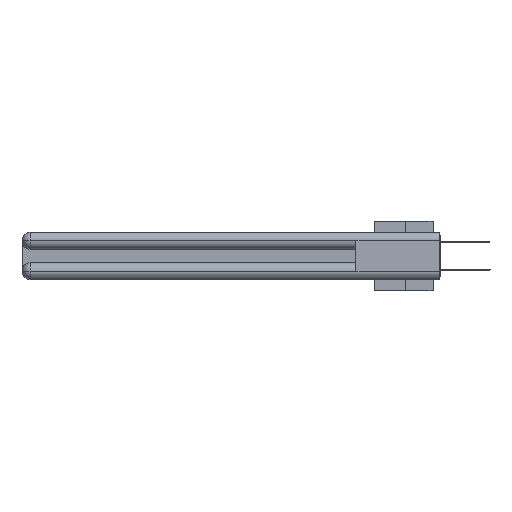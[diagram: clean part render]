
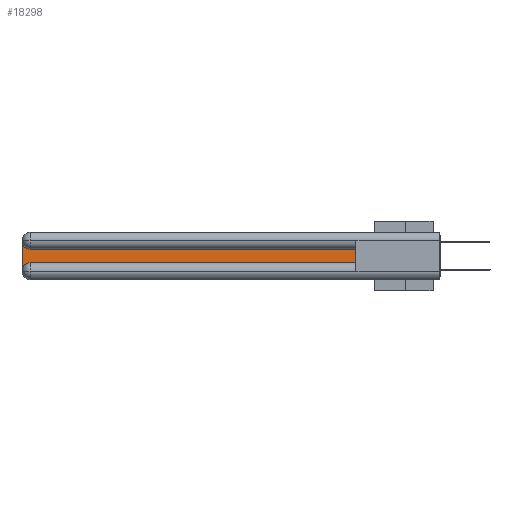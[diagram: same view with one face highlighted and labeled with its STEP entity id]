
A CAD part, left-side view. The second image highlights one B-rep face of the part: STEP entity #18298.
In plain terms, the highlighted planar face has unit normal (-1, 0, 0).
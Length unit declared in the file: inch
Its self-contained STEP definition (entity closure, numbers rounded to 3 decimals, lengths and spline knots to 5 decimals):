
#642 = CARTESIAN_POINT ( 'NONE',  ( 0.075, 2.94, -0.2775 ) ) ;
#2423 = AXIS2_PLACEMENT_3D ( 'NONE', #642, #32733, #19768 ) ;
#3171 = CIRCLE ( 'NONE', #18627, 0.06 ) ;
#3222 = CARTESIAN_POINT ( 'NONE',  ( 0.075, 3., -0.2775 ) ) ;
#3349 = FACE_OUTER_BOUND ( 'NONE', #8569, .T. ) ;
#5803 = ORIENTED_EDGE ( 'NONE', *, *, #13437, .T. ) ;
#7618 = CARTESIAN_POINT ( 'NONE',  ( 0.075, 0.6, -0.1225 ) ) ;
#7773 = DIRECTION ( 'NONE',  ( 0., -1., 0. ) ) ;
#8027 = CARTESIAN_POINT ( 'NONE',  ( 0.075, 2.94, -0.2175 ) ) ;
#8569 = EDGE_LOOP ( 'NONE', ( #12428, #5803, #15014, #15845, #37304, #25735 ) ) ;
#9439 = CARTESIAN_POINT ( 'NONE',  ( 0.075, 2.94, -0.1225 ) ) ;
#10481 = VERTEX_POINT ( 'NONE', #13727 ) ;
#10605 = LINE ( 'NONE', #32806, #41293 ) ;
#11036 = EDGE_CURVE ( 'NONE', #21050, #21309, #27271, .T. ) ;
#11140 = VECTOR ( 'NONE', #18580, 39.37008 ) ;
#11654 = EDGE_CURVE ( 'NONE', #21309, #23162, #41462, .T. ) ;
#12123 = EDGE_CURVE ( 'NONE', #38952, #21050, #24563, .T. ) ;
#12428 = ORIENTED_EDGE ( 'NONE', *, *, #15713, .T. ) ;
#12832 = PLANE ( 'NONE',  #30188 ) ;
#13394 = VECTOR ( 'NONE', #28221, 39.37008 ) ;
#13437 = EDGE_CURVE ( 'NONE', #41104, #10481, #3171, .T. ) ;
#13727 = CARTESIAN_POINT ( 'NONE',  ( 0.075, 3., -0.0625 ) ) ;
#15014 = ORIENTED_EDGE ( 'NONE', *, *, #33773, .T. ) ;
#15133 = VECTOR ( 'NONE', #7773, 39.37008 ) ;
#15713 = EDGE_CURVE ( 'NONE', #23162, #41104, #16065, .T. ) ;
#15845 = ORIENTED_EDGE ( 'NONE', *, *, #12123, .T. ) ;
#16065 = LINE ( 'NONE', #19632, #13394 ) ;
#16271 = DIRECTION ( 'NONE',  ( 0., 0., -1. ) ) ;
#18298 = ADVANCED_FACE ( 'NONE', ( #3349 ), #12832, .F. ) ;
#18580 = DIRECTION ( 'NONE',  ( 0., 0., 1. ) ) ;
#18627 = AXIS2_PLACEMENT_3D ( 'NONE', #19720, #31667, #35241 ) ;
#19632 = CARTESIAN_POINT ( 'NONE',  ( 0.075, 0.6, -0.1225 ) ) ;
#19720 = CARTESIAN_POINT ( 'NONE',  ( 0.075, 2.94, -0.0625 ) ) ;
#19768 = DIRECTION ( 'NONE',  ( 0., 0., -1. ) ) ;
#21050 = VERTEX_POINT ( 'NONE', #8027 ) ;
#21309 = VERTEX_POINT ( 'NONE', #31502 ) ;
#23162 = VERTEX_POINT ( 'NONE', #7618 ) ;
#24563 = CIRCLE ( 'NONE', #2423, 0.06 ) ;
#25597 = DIRECTION ( 'NONE',  ( 1., 0., 0. ) ) ;
#25735 = ORIENTED_EDGE ( 'NONE', *, *, #11654, .T. ) ;
#25810 = DIRECTION ( 'NONE',  ( 0., 0., -1. ) ) ;
#27271 = LINE ( 'NONE', #36316, #15133 ) ;
#28221 = DIRECTION ( 'NONE',  ( 0., 1., 0. ) ) ;
#28950 = CARTESIAN_POINT ( 'NONE',  ( 0.075, 3., -0.1225 ) ) ;
#30188 = AXIS2_PLACEMENT_3D ( 'NONE', #28950, #25597, #25810 ) ;
#31502 = CARTESIAN_POINT ( 'NONE',  ( 0.075, 0.6, -0.2175 ) ) ;
#31667 = DIRECTION ( 'NONE',  ( 1., 0., 0. ) ) ;
#32733 = DIRECTION ( 'NONE',  ( 1., 0., 0. ) ) ;
#32806 = CARTESIAN_POINT ( 'NONE',  ( 0.075, 3., -0.2175 ) ) ;
#33773 = EDGE_CURVE ( 'NONE', #10481, #38952, #10605, .T. ) ;
#35241 = DIRECTION ( 'NONE',  ( 0., 0., -1. ) ) ;
#35330 = CARTESIAN_POINT ( 'NONE',  ( 0.075, 0.6, -0.2175 ) ) ;
#36316 = CARTESIAN_POINT ( 'NONE',  ( 0.075, 0.6, -0.2175 ) ) ;
#37304 = ORIENTED_EDGE ( 'NONE', *, *, #11036, .T. ) ;
#38952 = VERTEX_POINT ( 'NONE', #3222 ) ;
#41104 = VERTEX_POINT ( 'NONE', #9439 ) ;
#41293 = VECTOR ( 'NONE', #16271, 39.37008 ) ;
#41462 = LINE ( 'NONE', #35330, #11140 ) ;
